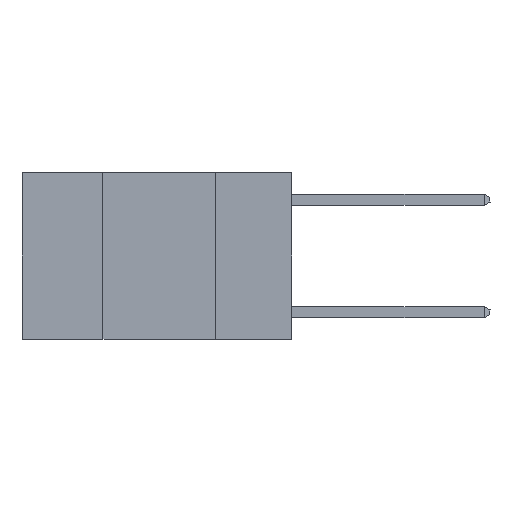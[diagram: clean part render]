
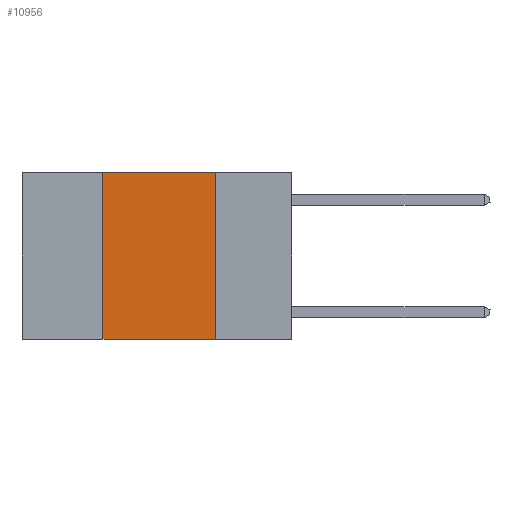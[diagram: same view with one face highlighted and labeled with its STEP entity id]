
A CAD part, left-side view. The second image highlights one B-rep face of the part: STEP entity #10956.
In plain terms, the highlighted planar face has unit normal (-1, 0, 0).
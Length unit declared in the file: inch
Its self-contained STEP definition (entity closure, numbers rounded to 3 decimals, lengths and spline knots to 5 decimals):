
#130 = DIRECTION ( 'NONE',  ( 0., 0., -1. ) ) ;
#1160 = ORIENTED_EDGE ( 'NONE', *, *, #17050, .F. ) ;
#2806 = DIRECTION ( 'NONE',  ( 0., -1., 0. ) ) ;
#3525 = LINE ( 'NONE', #26972, #7628 ) ;
#3699 = DIRECTION ( 'NONE',  ( 0., 0., -1. ) ) ;
#3828 = VECTOR ( 'NONE', #2806, 39.37008 ) ;
#5625 = DIRECTION ( 'NONE',  ( 0., -1., 0. ) ) ;
#5830 = CARTESIAN_POINT ( 'NONE',  ( 0., 0.6, 0. ) ) ;
#6239 = CARTESIAN_POINT ( 'NONE',  ( 0., 0.42, 0. ) ) ;
#7628 = VECTOR ( 'NONE', #11763, 39.37008 ) ;
#9203 = VERTEX_POINT ( 'NONE', #27372 ) ;
#9588 = VERTEX_POINT ( 'NONE', #27194 ) ;
#9740 = CARTESIAN_POINT ( 'NONE',  ( 0., 0.6, -0.37 ) ) ;
#10956 = ADVANCED_FACE ( 'NONE', ( #19022 ), #16461, .F. ) ;
#11409 = EDGE_CURVE ( 'NONE', #9588, #23491, #3525, .T. ) ;
#11763 = DIRECTION ( 'NONE',  ( 0., 0., 1. ) ) ;
#12934 = LINE ( 'NONE', #17608, #18207 ) ;
#13475 = ORIENTED_EDGE ( 'NONE', *, *, #27369, .F. ) ;
#14134 = LINE ( 'NONE', #9740, #21015 ) ;
#16140 = CARTESIAN_POINT ( 'NONE',  ( 0., 0.6, 0. ) ) ;
#16461 = PLANE ( 'NONE',  #21218 ) ;
#17050 = EDGE_CURVE ( 'NONE', #21530, #9203, #12934, .T. ) ;
#17608 = CARTESIAN_POINT ( 'NONE',  ( 0., 0.17, 0. ) ) ;
#17820 = ORIENTED_EDGE ( 'NONE', *, *, #11409, .F. ) ;
#18207 = VECTOR ( 'NONE', #130, 39.37008 ) ;
#18513 = ORIENTED_EDGE ( 'NONE', *, *, #26210, .T. ) ;
#19022 = FACE_OUTER_BOUND ( 'NONE', #20108, .T. ) ;
#19673 = CARTESIAN_POINT ( 'NONE',  ( 0., 0.17, 0. ) ) ;
#19989 = LINE ( 'NONE', #16140, #3828 ) ;
#20108 = EDGE_LOOP ( 'NONE', ( #1160, #13475, #17820, #18513 ) ) ;
#21015 = VECTOR ( 'NONE', #5625, 39.37008 ) ;
#21218 = AXIS2_PLACEMENT_3D ( 'NONE', #5830, #23144, #3699 ) ;
#21530 = VERTEX_POINT ( 'NONE', #19673 ) ;
#23144 = DIRECTION ( 'NONE',  ( 1., 0., 0. ) ) ;
#23491 = VERTEX_POINT ( 'NONE', #6239 ) ;
#26210 = EDGE_CURVE ( 'NONE', #9588, #9203, #14134, .T. ) ;
#26972 = CARTESIAN_POINT ( 'NONE',  ( 0., 0.42, 0. ) ) ;
#27194 = CARTESIAN_POINT ( 'NONE',  ( 0., 0.42, -0.37 ) ) ;
#27369 = EDGE_CURVE ( 'NONE', #23491, #21530, #19989, .T. ) ;
#27372 = CARTESIAN_POINT ( 'NONE',  ( 0., 0.17, -0.37 ) ) ;
